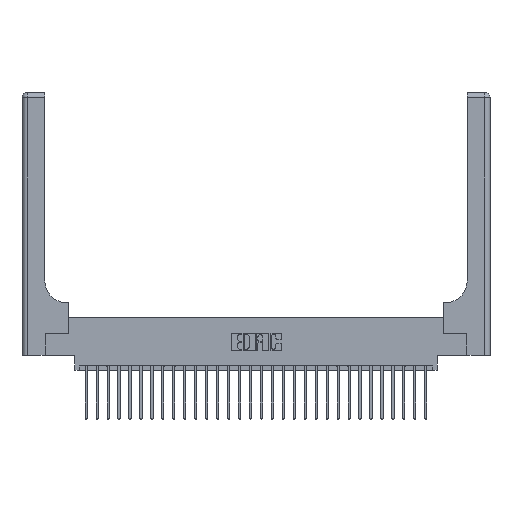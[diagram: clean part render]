
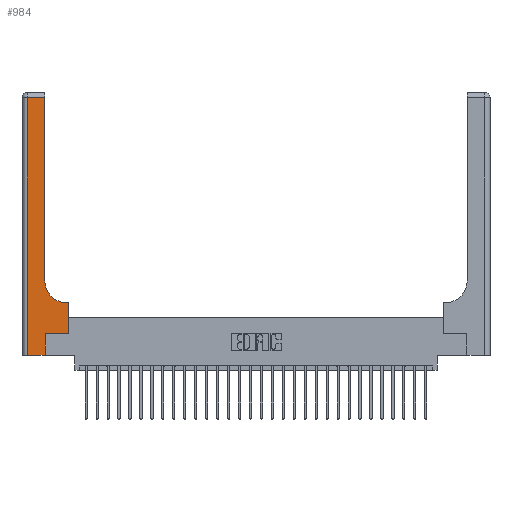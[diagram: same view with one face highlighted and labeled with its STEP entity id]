
A CAD part, top view. The second image highlights one B-rep face of the part: STEP entity #984.
In plain terms, the highlighted planar face has unit normal (0, 0, 1).
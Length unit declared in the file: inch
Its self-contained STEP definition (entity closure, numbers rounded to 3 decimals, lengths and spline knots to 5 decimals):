
#646 = LINE ( 'NONE', #9309, #2714 ) ;
#839 = EDGE_CURVE ( 'NONE', #8272, #2967, #19342, .T. ) ;
#984 = ADVANCED_FACE ( 'NONE', ( #26985 ), #16087, .F. ) ;
#1092 = ORIENTED_EDGE ( 'NONE', *, *, #18241, .T. ) ;
#1436 = ORIENTED_EDGE ( 'NONE', *, *, #23494, .T. ) ;
#1498 = CARTESIAN_POINT ( 'NONE',  ( 0.26, 3., 0.37 ) ) ;
#1803 = LINE ( 'NONE', #16704, #9909 ) ;
#2714 = VECTOR ( 'NONE', #8888, 39.37008 ) ;
#2967 = VERTEX_POINT ( 'NONE', #22066 ) ;
#3545 = CARTESIAN_POINT ( 'NONE',  ( 0., 2.94, 0.37 ) ) ;
#4571 = VERTEX_POINT ( 'NONE', #16251 ) ;
#4677 = ORIENTED_EDGE ( 'NONE', *, *, #10761, .T. ) ;
#4819 = CARTESIAN_POINT ( 'NONE',  ( 0.51, 0.85, 0.37 ) ) ;
#5740 = LINE ( 'NONE', #1498, #6133 ) ;
#5762 = VECTOR ( 'NONE', #5771, 39.37008 ) ;
#5771 = DIRECTION ( 'NONE',  ( 0., -1., 0. ) ) ;
#5817 = CARTESIAN_POINT ( 'NONE',  ( 0.26, 2.94, 0.37 ) ) ;
#5852 = EDGE_CURVE ( 'NONE', #21365, #4571, #646, .T. ) ;
#6133 = VECTOR ( 'NONE', #10031, 39.37008 ) ;
#6603 = EDGE_CURVE ( 'NONE', #12278, #10424, #19708, .T. ) ;
#7116 = EDGE_CURVE ( 'NONE', #13836, #12278, #5740, .T. ) ;
#7663 = DIRECTION ( 'NONE',  ( -1., 0., 0. ) ) ;
#7759 = CARTESIAN_POINT ( 'NONE',  ( 0.26, 0.6, 0.37 ) ) ;
#8272 = VERTEX_POINT ( 'NONE', #16299 ) ;
#8746 = CARTESIAN_POINT ( 'NONE',  ( 0.528, 0.25, 0.37 ) ) ;
#8888 = DIRECTION ( 'NONE',  ( 0., 1., 0. ) ) ;
#9309 = CARTESIAN_POINT ( 'NONE',  ( 0.528, 0.25, 0.37 ) ) ;
#9657 = LINE ( 'NONE', #22925, #21803 ) ;
#9782 = VERTEX_POINT ( 'NONE', #11749 ) ;
#9909 = VECTOR ( 'NONE', #19372, 39.37008 ) ;
#10031 = DIRECTION ( 'NONE',  ( 0., 1., 0. ) ) ;
#10424 = VERTEX_POINT ( 'NONE', #23966 ) ;
#10761 = EDGE_CURVE ( 'NONE', #2967, #21365, #1803, .T. ) ;
#11378 = DIRECTION ( 'NONE',  ( 0., 0., -1. ) ) ;
#11628 = CARTESIAN_POINT ( 'NONE',  ( 0.26, 0.85, 0.37 ) ) ;
#11749 = CARTESIAN_POINT ( 'NONE',  ( 0.06, 0., 0.37 ) ) ;
#12278 = VERTEX_POINT ( 'NONE', #5817 ) ;
#12360 = DIRECTION ( 'NONE',  ( 1., 0., 0. ) ) ;
#12515 = AXIS2_PLACEMENT_3D ( 'NONE', #4819, #11378, #13083 ) ;
#13060 = ORIENTED_EDGE ( 'NONE', *, *, #839, .T. ) ;
#13083 = DIRECTION ( 'NONE',  ( 1., 0., 0. ) ) ;
#13836 = VERTEX_POINT ( 'NONE', #11628 ) ;
#14491 = AXIS2_PLACEMENT_3D ( 'NONE', #18333, #15942, #26539 ) ;
#15239 = DIRECTION ( 'NONE',  ( 0., 1., 0. ) ) ;
#15627 = CARTESIAN_POINT ( 'NONE',  ( 0.51, 0.6, 0.37 ) ) ;
#15942 = DIRECTION ( 'NONE',  ( 0., 0., -1. ) ) ;
#16087 = PLANE ( 'NONE',  #14491 ) ;
#16251 = CARTESIAN_POINT ( 'NONE',  ( 0.528, 0.6, 0.37 ) ) ;
#16293 = LINE ( 'NONE', #26906, #5762 ) ;
#16299 = CARTESIAN_POINT ( 'NONE',  ( 0.265, 0., 0.37 ) ) ;
#16704 = CARTESIAN_POINT ( 'NONE',  ( 0.265, 0.25, 0.37 ) ) ;
#17151 = ORIENTED_EDGE ( 'NONE', *, *, #7116, .T. ) ;
#17324 = VECTOR ( 'NONE', #22887, 39.37008 ) ;
#17763 = VERTEX_POINT ( 'NONE', #15627 ) ;
#18241 = EDGE_CURVE ( 'NONE', #4571, #17763, #23178, .T. ) ;
#18333 = CARTESIAN_POINT ( 'NONE',  ( 0., 3., 0.37 ) ) ;
#19342 = LINE ( 'NONE', #25850, #24809 ) ;
#19372 = DIRECTION ( 'NONE',  ( 1., 0., 0. ) ) ;
#19450 = EDGE_CURVE ( 'NONE', #9782, #8272, #9657, .T. ) ;
#19708 = LINE ( 'NONE', #3545, #26115 ) ;
#21365 = VERTEX_POINT ( 'NONE', #8746 ) ;
#21515 = CIRCLE ( 'NONE', #12515, 0.25 ) ;
#21679 = EDGE_LOOP ( 'NONE', ( #17151, #26464, #22391, #23421, #13060, #4677, #21864, #1092, #1436 ) ) ;
#21803 = VECTOR ( 'NONE', #12360, 39.37008 ) ;
#21864 = ORIENTED_EDGE ( 'NONE', *, *, #5852, .T. ) ;
#22066 = CARTESIAN_POINT ( 'NONE',  ( 0.265, 0.25, 0.37 ) ) ;
#22391 = ORIENTED_EDGE ( 'NONE', *, *, #25715, .T. ) ;
#22887 = DIRECTION ( 'NONE',  ( -1., 0., 0. ) ) ;
#22925 = CARTESIAN_POINT ( 'NONE',  ( 0., 0., 0.37 ) ) ;
#23178 = LINE ( 'NONE', #7759, #17324 ) ;
#23421 = ORIENTED_EDGE ( 'NONE', *, *, #19450, .T. ) ;
#23494 = EDGE_CURVE ( 'NONE', #17763, #13836, #21515, .T. ) ;
#23966 = CARTESIAN_POINT ( 'NONE',  ( 0.06, 2.94, 0.37 ) ) ;
#24809 = VECTOR ( 'NONE', #15239, 39.37008 ) ;
#25715 = EDGE_CURVE ( 'NONE', #10424, #9782, #16293, .T. ) ;
#25850 = CARTESIAN_POINT ( 'NONE',  ( 0.265, 0., 0.37 ) ) ;
#26115 = VECTOR ( 'NONE', #7663, 39.37008 ) ;
#26464 = ORIENTED_EDGE ( 'NONE', *, *, #6603, .T. ) ;
#26539 = DIRECTION ( 'NONE',  ( -1., 0., 0. ) ) ;
#26906 = CARTESIAN_POINT ( 'NONE',  ( 0.06, 3., 0.37 ) ) ;
#26985 = FACE_OUTER_BOUND ( 'NONE', #21679, .T. ) ;
